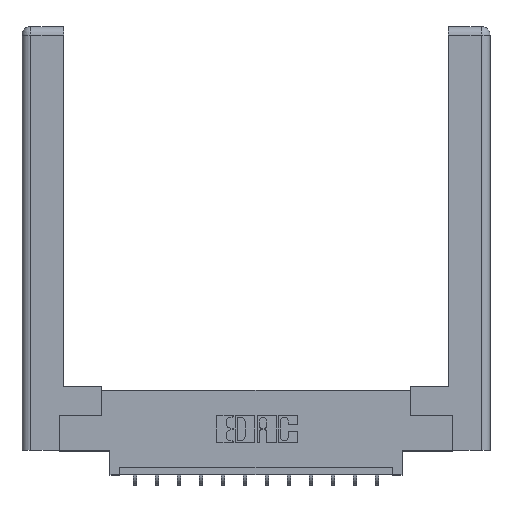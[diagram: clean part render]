
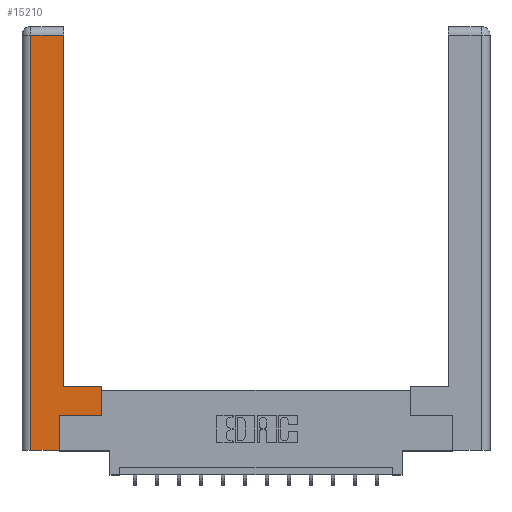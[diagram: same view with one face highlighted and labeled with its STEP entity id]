
A CAD part, top view. The second image highlights one B-rep face of the part: STEP entity #15210.
In plain terms, the highlighted planar face has unit normal (0, 0, 1).
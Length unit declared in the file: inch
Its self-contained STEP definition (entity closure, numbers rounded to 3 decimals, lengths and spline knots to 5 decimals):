
#181 = CARTESIAN_POINT ( 'NONE',  ( 0.565, 0.245, 0. ) ) ;
#193 = VECTOR ( 'NONE', #2213, 39.37008 ) ;
#511 = VECTOR ( 'NONE', #4687, 39.37008 ) ;
#931 = ORIENTED_EDGE ( 'NONE', *, *, #4737, .T. ) ;
#933 = VECTOR ( 'NONE', #12798, 39.37008 ) ;
#1021 = EDGE_CURVE ( 'NONE', #7247, #12092, #8848, .T. ) ;
#1034 = CARTESIAN_POINT ( 'NONE',  ( 0.565, 0.45, 0. ) ) ;
#1474 = LINE ( 'NONE', #13978, #933 ) ;
#1502 = VECTOR ( 'NONE', #4578, 39.37008 ) ;
#1555 = EDGE_CURVE ( 'NONE', #10537, #13205, #1474, .T. ) ;
#2213 = DIRECTION ( 'NONE',  ( 1., 0., 0. ) ) ;
#2220 = CARTESIAN_POINT ( 'NONE',  ( 0.265, 0.245, 0. ) ) ;
#2419 = VERTEX_POINT ( 'NONE', #4898 ) ;
#2436 = DIRECTION ( 'NONE',  ( 0., 1., 0. ) ) ;
#2579 = VECTOR ( 'NONE', #7513, 39.37008 ) ;
#2793 = VERTEX_POINT ( 'NONE', #13823 ) ;
#3303 = CARTESIAN_POINT ( 'NONE',  ( 0.295, 0.45, 0. ) ) ;
#3397 = LINE ( 'NONE', #14356, #7008 ) ;
#3539 = CARTESIAN_POINT ( 'NONE',  ( 0., 0., 0. ) ) ;
#4578 = DIRECTION ( 'NONE',  ( -1., 0., 0. ) ) ;
#4687 = DIRECTION ( 'NONE',  ( 0., 1., 0. ) ) ;
#4724 = PLANE ( 'NONE',  #15152 ) ;
#4731 = ORIENTED_EDGE ( 'NONE', *, *, #1021, .T. ) ;
#4737 = EDGE_CURVE ( 'NONE', #2419, #2793, #10113, .T. ) ;
#4781 = DIRECTION ( 'NONE',  ( 0., 0., -1. ) ) ;
#4898 = CARTESIAN_POINT ( 'NONE',  ( 0.265, 0., 0. ) ) ;
#5904 = DIRECTION ( 'NONE',  ( -1., 0., 0. ) ) ;
#6591 = CARTESIAN_POINT ( 'NONE',  ( 0.565, 0.245, 0. ) ) ;
#6920 = EDGE_CURVE ( 'NONE', #7308, #10537, #14970, .T. ) ;
#6934 = EDGE_LOOP ( 'NONE', ( #8436, #13848, #10924, #10979, #931, #9871, #14118, #4731 ) ) ;
#7008 = VECTOR ( 'NONE', #15472, 39.37008 ) ;
#7054 = DIRECTION ( 'NONE',  ( -1., 0., 0. ) ) ;
#7247 = VERTEX_POINT ( 'NONE', #1034 ) ;
#7308 = VERTEX_POINT ( 'NONE', #8970 ) ;
#7513 = DIRECTION ( 'NONE',  ( 1., 0., 0. ) ) ;
#8436 = ORIENTED_EDGE ( 'NONE', *, *, #15225, .T. ) ;
#8848 = LINE ( 'NONE', #3303, #1502 ) ;
#8970 = CARTESIAN_POINT ( 'NONE',  ( 0.295, 2.94, 0. ) ) ;
#9792 = CARTESIAN_POINT ( 'NONE',  ( 0.565, 0.45, 0. ) ) ;
#9871 = ORIENTED_EDGE ( 'NONE', *, *, #10807, .T. ) ;
#10113 = LINE ( 'NONE', #2220, #511 ) ;
#10510 = VERTEX_POINT ( 'NONE', #6591 ) ;
#10537 = VERTEX_POINT ( 'NONE', #12858 ) ;
#10807 = EDGE_CURVE ( 'NONE', #2793, #10510, #14721, .T. ) ;
#10924 = ORIENTED_EDGE ( 'NONE', *, *, #1555, .T. ) ;
#10979 = ORIENTED_EDGE ( 'NONE', *, *, #15612, .T. ) ;
#11733 = VECTOR ( 'NONE', #7054, 39.37008 ) ;
#12092 = VERTEX_POINT ( 'NONE', #12484 ) ;
#12112 = CARTESIAN_POINT ( 'NONE',  ( 0.0615, 2.94, 0. ) ) ;
#12484 = CARTESIAN_POINT ( 'NONE',  ( 0.295, 0.45, 0. ) ) ;
#12798 = DIRECTION ( 'NONE',  ( 0., -1., 0. ) ) ;
#12858 = CARTESIAN_POINT ( 'NONE',  ( 0.0615, 2.94, 0. ) ) ;
#13074 = LINE ( 'NONE', #9792, #15381 ) ;
#13205 = VERTEX_POINT ( 'NONE', #15101 ) ;
#13437 = FACE_OUTER_BOUND ( 'NONE', #6934, .T. ) ;
#13613 = LINE ( 'NONE', #14476, #193 ) ;
#13689 = EDGE_CURVE ( 'NONE', #10510, #7247, #13074, .T. ) ;
#13823 = CARTESIAN_POINT ( 'NONE',  ( 0.265, 0.245, 0. ) ) ;
#13848 = ORIENTED_EDGE ( 'NONE', *, *, #6920, .T. ) ;
#13978 = CARTESIAN_POINT ( 'NONE',  ( 0.0615, 0., 0. ) ) ;
#14118 = ORIENTED_EDGE ( 'NONE', *, *, #13689, .T. ) ;
#14356 = CARTESIAN_POINT ( 'NONE',  ( 0.295, 3., 0. ) ) ;
#14476 = CARTESIAN_POINT ( 'NONE',  ( 0.265, 0., 0. ) ) ;
#14721 = LINE ( 'NONE', #181, #2579 ) ;
#14970 = LINE ( 'NONE', #12112, #11733 ) ;
#15101 = CARTESIAN_POINT ( 'NONE',  ( 0.0615, 0., 0. ) ) ;
#15152 = AXIS2_PLACEMENT_3D ( 'NONE', #3539, #4781, #5904 ) ;
#15210 = ADVANCED_FACE ( 'NONE', ( #13437 ), #4724, .F. ) ;
#15225 = EDGE_CURVE ( 'NONE', #12092, #7308, #3397, .T. ) ;
#15381 = VECTOR ( 'NONE', #2436, 39.37008 ) ;
#15472 = DIRECTION ( 'NONE',  ( 0., 1., 0. ) ) ;
#15612 = EDGE_CURVE ( 'NONE', #13205, #2419, #13613, .T. ) ;
